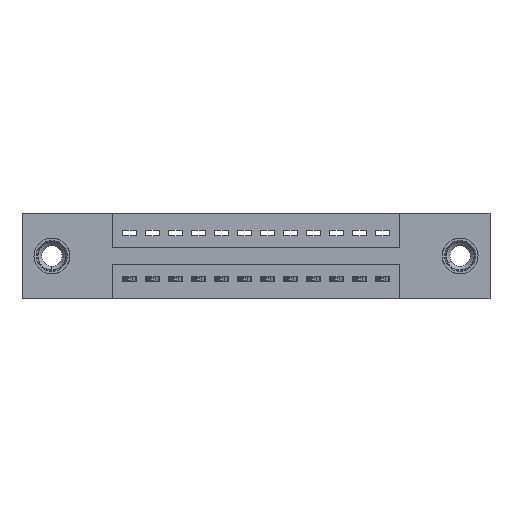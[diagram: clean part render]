
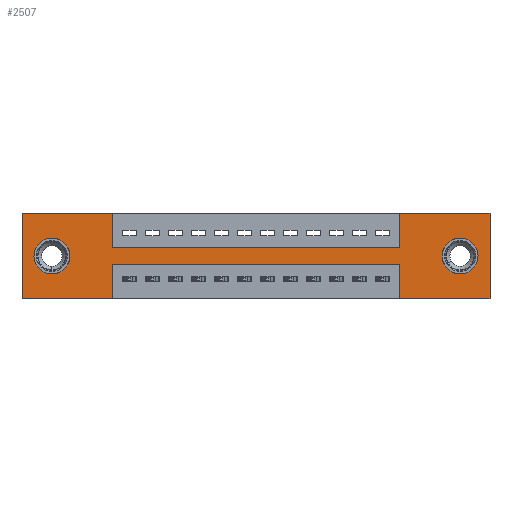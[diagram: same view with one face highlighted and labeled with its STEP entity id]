
A CAD part, front view. The second image highlights one B-rep face of the part: STEP entity #2507.
In plain terms, the highlighted planar face has unit normal (0, -1, 0).
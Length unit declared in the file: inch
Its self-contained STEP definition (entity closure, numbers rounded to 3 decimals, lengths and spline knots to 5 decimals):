
#56 = ORIENTED_EDGE ( 'NONE', *, *, #13348, .F. ) ;
#57 = CARTESIAN_POINT ( 'NONE',  ( 0.3925, 0., -0.22 ) ) ;
#144 = CARTESIAN_POINT ( 'NONE',  ( 0.3925, 0., -0.15 ) ) ;
#160 = LINE ( 'NONE', #57, #8591 ) ;
#226 = DIRECTION ( 'NONE',  ( -1., 0., 0. ) ) ;
#264 = CARTESIAN_POINT ( 'NONE',  ( 1.6425, 0., -0.37 ) ) ;
#269 = ORIENTED_EDGE ( 'NONE', *, *, #13231, .T. ) ;
#271 = DIRECTION ( 'NONE',  ( 1., 0., 0. ) ) ;
#516 = EDGE_CURVE ( 'NONE', #3126, #5865, #6321, .T. ) ;
#576 = DIRECTION ( 'NONE',  ( 0., -1., 0. ) ) ;
#652 = VERTEX_POINT ( 'NONE', #7140 ) ;
#664 = LINE ( 'NONE', #6834, #12078 ) ;
#673 = CARTESIAN_POINT ( 'NONE',  ( 0.3925, 0., -0.15 ) ) ;
#698 = CARTESIAN_POINT ( 'NONE',  ( 1.6425, 0., -0.15 ) ) ;
#1090 = EDGE_CURVE ( 'NONE', #13553, #10937, #1844, .T. ) ;
#1098 = CARTESIAN_POINT ( 'NONE',  ( 0., 0., 0. ) ) ;
#1233 = DIRECTION ( 'NONE',  ( 0., 0., 1. ) ) ;
#1302 = CARTESIAN_POINT ( 'NONE',  ( 1.6425, 0., 0. ) ) ;
#1452 = CARTESIAN_POINT ( 'NONE',  ( 0.13, 0., -0.107 ) ) ;
#1464 = DIRECTION ( 'NONE',  ( 1., 0., 0. ) ) ;
#1650 = CIRCLE ( 'NONE', #7011, 0.078 ) ;
#1773 = VERTEX_POINT ( 'NONE', #4098 ) ;
#1844 = LINE ( 'NONE', #10827, #2599 ) ;
#1993 = ORIENTED_EDGE ( 'NONE', *, *, #12646, .F. ) ;
#2065 = CARTESIAN_POINT ( 'NONE',  ( 0.3925, 0., -0.37 ) ) ;
#2145 = EDGE_CURVE ( 'NONE', #5865, #11055, #12613, .T. ) ;
#2223 = CARTESIAN_POINT ( 'NONE',  ( 0.13, 0., -0.185 ) ) ;
#2507 = ADVANCED_FACE ( 'NONE', ( #8690, #5799, #11452 ), #8593, .T. ) ;
#2599 = VECTOR ( 'NONE', #1464, 39.37008 ) ;
#2925 = ORIENTED_EDGE ( 'NONE', *, *, #13035, .F. ) ;
#2973 = LINE ( 'NONE', #264, #8555 ) ;
#2999 = DIRECTION ( 'NONE',  ( 0., 0., -1. ) ) ;
#3126 = VERTEX_POINT ( 'NONE', #673 ) ;
#3177 = VERTEX_POINT ( 'NONE', #8676 ) ;
#3358 = VECTOR ( 'NONE', #8749, 39.37008 ) ;
#3390 = EDGE_CURVE ( 'NONE', #6161, #8088, #664, .T. ) ;
#3410 = DIRECTION ( 'NONE',  ( 0., 0., 1. ) ) ;
#3462 = ORIENTED_EDGE ( 'NONE', *, *, #5198, .F. ) ;
#3591 = AXIS2_PLACEMENT_3D ( 'NONE', #13250, #6950, #14278 ) ;
#3722 = LINE ( 'NONE', #7705, #3358 ) ;
#4082 = CIRCLE ( 'NONE', #6638, 0.078 ) ;
#4098 = CARTESIAN_POINT ( 'NONE',  ( 2.035, 0., -0.37 ) ) ;
#4391 = EDGE_LOOP ( 'NONE', ( #5069, #1993, #56, #2925, #10607, #13056, #10291, #9952, #12403, #6474, #3462, #8968 ) ) ;
#4396 = CARTESIAN_POINT ( 'NONE',  ( 1.905, 0., -0.107 ) ) ;
#4407 = LINE ( 'NONE', #2065, #7422 ) ;
#4408 = CARTESIAN_POINT ( 'NONE',  ( 1.6425, 0., -0.37 ) ) ;
#5020 = VERTEX_POINT ( 'NONE', #5333 ) ;
#5069 = ORIENTED_EDGE ( 'NONE', *, *, #11939, .F. ) ;
#5081 = DIRECTION ( 'NONE',  ( 0., 0., -1. ) ) ;
#5198 = EDGE_CURVE ( 'NONE', #8088, #13553, #6422, .T. ) ;
#5333 = CARTESIAN_POINT ( 'NONE',  ( 0.3925, 0., -0.22 ) ) ;
#5353 = CARTESIAN_POINT ( 'NONE',  ( 0., 0., 0. ) ) ;
#5414 = ORIENTED_EDGE ( 'NONE', *, *, #11999, .T. ) ;
#5799 = FACE_BOUND ( 'NONE', #9259, .T. ) ;
#5865 = VERTEX_POINT ( 'NONE', #698 ) ;
#5885 = CARTESIAN_POINT ( 'NONE',  ( 0.3925, 0., -0.37 ) ) ;
#6161 = VERTEX_POINT ( 'NONE', #5885 ) ;
#6268 = VERTEX_POINT ( 'NONE', #1452 ) ;
#6321 = LINE ( 'NONE', #144, #11933 ) ;
#6373 = DIRECTION ( 'NONE',  ( 0., 1., 0. ) ) ;
#6412 = VECTOR ( 'NONE', #12099, 39.37008 ) ;
#6422 = LINE ( 'NONE', #10919, #11370 ) ;
#6425 = EDGE_CURVE ( 'NONE', #13081, #11561, #8094, .T. ) ;
#6474 = ORIENTED_EDGE ( 'NONE', *, *, #1090, .F. ) ;
#6638 = AXIS2_PLACEMENT_3D ( 'NONE', #2223, #9953, #3410 ) ;
#6834 = CARTESIAN_POINT ( 'NONE',  ( 0., 0., -0.37 ) ) ;
#6950 = DIRECTION ( 'NONE',  ( 0., 1., 0. ) ) ;
#6970 = DIRECTION ( 'NONE',  ( 0., 1., 0. ) ) ;
#7011 = AXIS2_PLACEMENT_3D ( 'NONE', #13269, #6970, #14296 ) ;
#7140 = CARTESIAN_POINT ( 'NONE',  ( 2.035, 0., 0. ) ) ;
#7262 = VECTOR ( 'NONE', #2999, 39.37008 ) ;
#7422 = VECTOR ( 'NONE', #8770, 39.37008 ) ;
#7520 = ORIENTED_EDGE ( 'NONE', *, *, #6425, .T. ) ;
#7552 = CARTESIAN_POINT ( 'NONE',  ( 0.3925, 0., 0. ) ) ;
#7699 = VECTOR ( 'NONE', #8030, 39.37008 ) ;
#7705 = CARTESIAN_POINT ( 'NONE',  ( 0., 0., -0.37 ) ) ;
#8030 = DIRECTION ( 'NONE',  ( 0., 0., -1. ) ) ;
#8088 = VERTEX_POINT ( 'NONE', #11312 ) ;
#8094 = CIRCLE ( 'NONE', #10337, 0.078 ) ;
#8461 = VERTEX_POINT ( 'NONE', #4408 ) ;
#8555 = VECTOR ( 'NONE', #12386, 39.37008 ) ;
#8591 = VECTOR ( 'NONE', #226, 39.37008 ) ;
#8593 = PLANE ( 'NONE',  #9241 ) ;
#8608 = CARTESIAN_POINT ( 'NONE',  ( 0., 0., -0.37 ) ) ;
#8676 = CARTESIAN_POINT ( 'NONE',  ( 0.13, 0., -0.263 ) ) ;
#8690 = FACE_BOUND ( 'NONE', #11966, .T. ) ;
#8749 = DIRECTION ( 'NONE',  ( -1., 0., 0. ) ) ;
#8770 = DIRECTION ( 'NONE',  ( 0., 0., -1. ) ) ;
#8837 = EDGE_CURVE ( 'NONE', #652, #1773, #13245, .T. ) ;
#8861 = VERTEX_POINT ( 'NONE', #13268 ) ;
#8968 = ORIENTED_EDGE ( 'NONE', *, *, #3390, .F. ) ;
#8970 = DIRECTION ( 'NONE',  ( -1., 0., 0. ) ) ;
#9241 = AXIS2_PLACEMENT_3D ( 'NONE', #8608, #576, #5081 ) ;
#9242 = LINE ( 'NONE', #1098, #6412 ) ;
#9259 = EDGE_LOOP ( 'NONE', ( #269, #5414 ) ) ;
#9453 = EDGE_CURVE ( 'NONE', #11561, #13081, #10288, .T. ) ;
#9595 = CARTESIAN_POINT ( 'NONE',  ( 0.3925, 0., 0. ) ) ;
#9834 = CARTESIAN_POINT ( 'NONE',  ( 1.6425, 0., 0. ) ) ;
#9841 = VECTOR ( 'NONE', #1233, 39.37008 ) ;
#9952 = ORIENTED_EDGE ( 'NONE', *, *, #516, .F. ) ;
#9953 = DIRECTION ( 'NONE',  ( 0., 1., 0. ) ) ;
#10199 = CARTESIAN_POINT ( 'NONE',  ( 1.905, 0., -0.263 ) ) ;
#10288 = CIRCLE ( 'NONE', #3591, 0.078 ) ;
#10291 = ORIENTED_EDGE ( 'NONE', *, *, #2145, .F. ) ;
#10337 = AXIS2_PLACEMENT_3D ( 'NONE', #12683, #6373, #13726 ) ;
#10607 = ORIENTED_EDGE ( 'NONE', *, *, #8837, .F. ) ;
#10827 = CARTESIAN_POINT ( 'NONE',  ( 0., 0., 0. ) ) ;
#10919 = CARTESIAN_POINT ( 'NONE',  ( 0., 0., 0. ) ) ;
#10937 = VERTEX_POINT ( 'NONE', #7552 ) ;
#11055 = VERTEX_POINT ( 'NONE', #9834 ) ;
#11171 = EDGE_CURVE ( 'NONE', #11055, #652, #9242, .T. ) ;
#11312 = CARTESIAN_POINT ( 'NONE',  ( 0., 0., -0.37 ) ) ;
#11370 = VECTOR ( 'NONE', #14030, 39.37008 ) ;
#11452 = FACE_OUTER_BOUND ( 'NONE', #4391, .T. ) ;
#11561 = VERTEX_POINT ( 'NONE', #10199 ) ;
#11933 = VECTOR ( 'NONE', #271, 39.37008 ) ;
#11939 = EDGE_CURVE ( 'NONE', #5020, #6161, #4407, .T. ) ;
#11966 = EDGE_LOOP ( 'NONE', ( #7520, #12083 ) ) ;
#11999 = EDGE_CURVE ( 'NONE', #3177, #6268, #4082, .T. ) ;
#12078 = VECTOR ( 'NONE', #8970, 39.37008 ) ;
#12083 = ORIENTED_EDGE ( 'NONE', *, *, #9453, .T. ) ;
#12099 = DIRECTION ( 'NONE',  ( 1., 0., 0. ) ) ;
#12380 = EDGE_CURVE ( 'NONE', #10937, #3126, #13149, .T. ) ;
#12386 = DIRECTION ( 'NONE',  ( 0., 0., 1. ) ) ;
#12403 = ORIENTED_EDGE ( 'NONE', *, *, #12380, .F. ) ;
#12613 = LINE ( 'NONE', #1302, #9841 ) ;
#12646 = EDGE_CURVE ( 'NONE', #8861, #5020, #160, .T. ) ;
#12683 = CARTESIAN_POINT ( 'NONE',  ( 1.905, 0., -0.185 ) ) ;
#13035 = EDGE_CURVE ( 'NONE', #1773, #8461, #3722, .T. ) ;
#13056 = ORIENTED_EDGE ( 'NONE', *, *, #11171, .F. ) ;
#13081 = VERTEX_POINT ( 'NONE', #4396 ) ;
#13149 = LINE ( 'NONE', #9595, #7262 ) ;
#13231 = EDGE_CURVE ( 'NONE', #6268, #3177, #1650, .T. ) ;
#13245 = LINE ( 'NONE', #14245, #7699 ) ;
#13250 = CARTESIAN_POINT ( 'NONE',  ( 1.905, 0., -0.185 ) ) ;
#13268 = CARTESIAN_POINT ( 'NONE',  ( 1.6425, 0., -0.22 ) ) ;
#13269 = CARTESIAN_POINT ( 'NONE',  ( 0.13, 0., -0.185 ) ) ;
#13348 = EDGE_CURVE ( 'NONE', #8461, #8861, #2973, .T. ) ;
#13553 = VERTEX_POINT ( 'NONE', #5353 ) ;
#13726 = DIRECTION ( 'NONE',  ( 0., 0., -1. ) ) ;
#14030 = DIRECTION ( 'NONE',  ( 0., 0., 1. ) ) ;
#14245 = CARTESIAN_POINT ( 'NONE',  ( 2.035, 0., 0. ) ) ;
#14278 = DIRECTION ( 'NONE',  ( 0., 0., -1. ) ) ;
#14296 = DIRECTION ( 'NONE',  ( 0., 0., 1. ) ) ;
